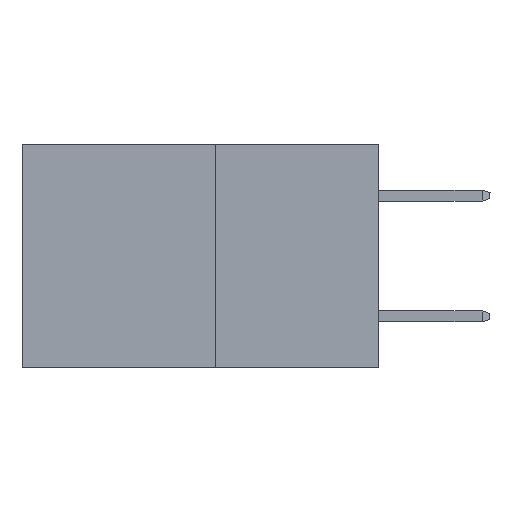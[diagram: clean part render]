
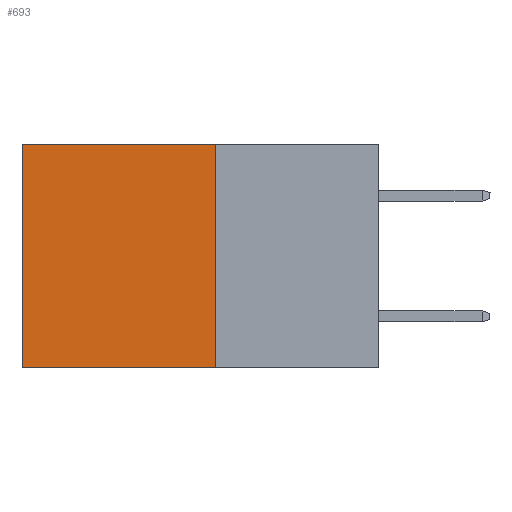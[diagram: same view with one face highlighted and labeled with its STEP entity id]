
A CAD part, left-side view. The second image highlights one B-rep face of the part: STEP entity #693.
In plain terms, the highlighted planar face has unit normal (-1, 0, 0).
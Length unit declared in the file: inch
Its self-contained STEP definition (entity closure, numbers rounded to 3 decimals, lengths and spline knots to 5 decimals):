
#692 = VERTEX_POINT ( 'NONE', #3618 ) ;
#693 = ADVANCED_FACE ( 'NONE', ( #4008 ), #3582, .F. ) ;
#1102 = VERTEX_POINT ( 'NONE', #6416 ) ;
#1171 = EDGE_CURVE ( 'NONE', #1102, #5211, #7964, .T. ) ;
#1451 = DIRECTION ( 'NONE',  ( 0., 1., 0. ) ) ;
#1787 = ORIENTED_EDGE ( 'NONE', *, *, #5940, .T. ) ;
#1796 = ORIENTED_EDGE ( 'NONE', *, *, #3505, .F. ) ;
#1808 = ORIENTED_EDGE ( 'NONE', *, *, #1171, .F. ) ;
#1818 = ORIENTED_EDGE ( 'NONE', *, *, #8330, .T. ) ;
#2488 = LINE ( 'NONE', #5510, #6677 ) ;
#2825 = DIRECTION ( 'NONE',  ( 0., 1., 0. ) ) ;
#3296 = VECTOR ( 'NONE', #1451, 39.37008 ) ;
#3301 = VERTEX_POINT ( 'NONE', #3500 ) ;
#3500 = CARTESIAN_POINT ( 'NONE',  ( 0.277, 0.59, 0. ) ) ;
#3505 = EDGE_CURVE ( 'NONE', #5211, #692, #7822, .T. ) ;
#3582 = PLANE ( 'NONE',  #4355 ) ;
#3597 = CARTESIAN_POINT ( 'NONE',  ( 0.277, 0.27, -0.37 ) ) ;
#3618 = CARTESIAN_POINT ( 'NONE',  ( 0.277, 0.59, -0.37 ) ) ;
#4008 = FACE_OUTER_BOUND ( 'NONE', #5860, .T. ) ;
#4066 = DIRECTION ( 'NONE',  ( 0., 0., -1. ) ) ;
#4113 = DIRECTION ( 'NONE',  ( 1., 0., 0. ) ) ;
#4231 = DIRECTION ( 'NONE',  ( 0., 0., -1. ) ) ;
#4355 = AXIS2_PLACEMENT_3D ( 'NONE', #3597, #4113, #4066 ) ;
#4401 = DIRECTION ( 'NONE',  ( 0., 0., -1. ) ) ;
#4911 = CARTESIAN_POINT ( 'NONE',  ( 0.277, 0.27, -0.37 ) ) ;
#5147 = CARTESIAN_POINT ( 'NONE',  ( 0.277, 0.27, -0.37 ) ) ;
#5211 = VERTEX_POINT ( 'NONE', #5736 ) ;
#5510 = CARTESIAN_POINT ( 'NONE',  ( 0.277, 0.59, -0.37 ) ) ;
#5667 = VECTOR ( 'NONE', #2825, 39.37008 ) ;
#5736 = CARTESIAN_POINT ( 'NONE',  ( 0.277, 0.27, -0.37 ) ) ;
#5840 = VECTOR ( 'NONE', #4231, 39.37008 ) ;
#5860 = EDGE_LOOP ( 'NONE', ( #1787, #1796, #1808, #1818 ) ) ;
#5940 = EDGE_CURVE ( 'NONE', #3301, #692, #2488, .T. ) ;
#6416 = CARTESIAN_POINT ( 'NONE',  ( 0.277, 0.27, 0. ) ) ;
#6677 = VECTOR ( 'NONE', #4401, 39.37008 ) ;
#7822 = LINE ( 'NONE', #4911, #5667 ) ;
#7964 = LINE ( 'NONE', #5147, #5840 ) ;
#8330 = EDGE_CURVE ( 'NONE', #1102, #3301, #9457, .T. ) ;
#8502 = CARTESIAN_POINT ( 'NONE',  ( 0.277, 0.27, 0. ) ) ;
#9457 = LINE ( 'NONE', #8502, #3296 ) ;
